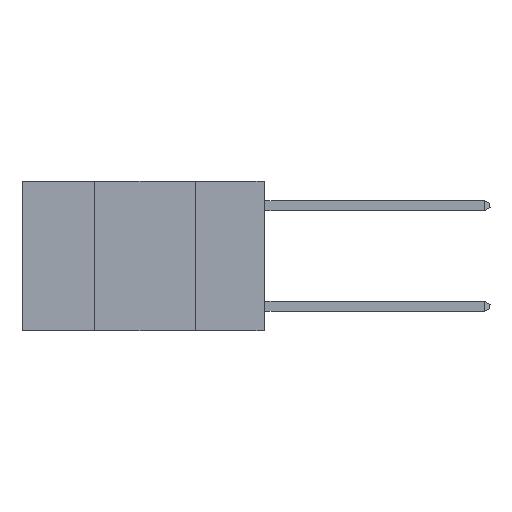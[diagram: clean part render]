
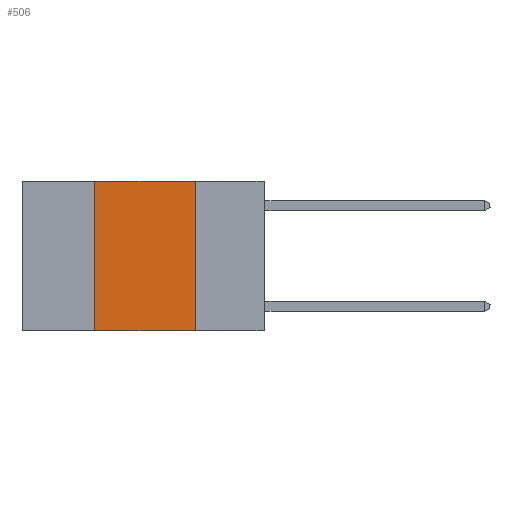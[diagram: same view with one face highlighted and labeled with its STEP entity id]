
A CAD part, left-side view. The second image highlights one B-rep face of the part: STEP entity #506.
In plain terms, the highlighted planar face has unit normal (-1, 0, 0).
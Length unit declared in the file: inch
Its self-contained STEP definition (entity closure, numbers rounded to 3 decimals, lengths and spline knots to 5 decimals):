
#87 = DIRECTION ( 'NONE',  ( 0., -1., 0. ) ) ;
#319 = CARTESIAN_POINT ( 'NONE',  ( 0., 0.42, 0. ) ) ;
#506 = ADVANCED_FACE ( 'NONE', ( #536 ), #17662, .F. ) ;
#536 = FACE_OUTER_BOUND ( 'NONE', #3672, .T. ) ;
#1416 = AXIS2_PLACEMENT_3D ( 'NONE', #10290, #12210, #27448 ) ;
#1519 = EDGE_CURVE ( 'NONE', #7277, #27388, #13245, .T. ) ;
#3672 = EDGE_LOOP ( 'NONE', ( #21942, #30267, #30392, #14577 ) ) ;
#4250 = EDGE_CURVE ( 'NONE', #27388, #6150, #17445, .T. ) ;
#4263 = LINE ( 'NONE', #23806, #19465 ) ;
#5405 = CARTESIAN_POINT ( 'NONE',  ( 0., 0.6, 0. ) ) ;
#6150 = VERTEX_POINT ( 'NONE', #16122 ) ;
#7277 = VERTEX_POINT ( 'NONE', #319 ) ;
#7963 = DIRECTION ( 'NONE',  ( 0., -1., 0. ) ) ;
#10290 = CARTESIAN_POINT ( 'NONE',  ( 0., 0.6, 0. ) ) ;
#12210 = DIRECTION ( 'NONE',  ( 1., 0., 0. ) ) ;
#12755 = CARTESIAN_POINT ( 'NONE',  ( 0., 0.42, -0.37 ) ) ;
#13245 = LINE ( 'NONE', #5405, #14941 ) ;
#13765 = VERTEX_POINT ( 'NONE', #12755 ) ;
#14577 = ORIENTED_EDGE ( 'NONE', *, *, #26245, .T. ) ;
#14941 = VECTOR ( 'NONE', #7963, 39.37008 ) ;
#16122 = CARTESIAN_POINT ( 'NONE',  ( 0., 0.17, -0.37 ) ) ;
#17062 = CARTESIAN_POINT ( 'NONE',  ( 0., 0.6, -0.37 ) ) ;
#17445 = LINE ( 'NONE', #22412, #21580 ) ;
#17662 = PLANE ( 'NONE',  #1416 ) ;
#19465 = VECTOR ( 'NONE', #28471, 39.37008 ) ;
#19943 = LINE ( 'NONE', #17062, #22525 ) ;
#21571 = CARTESIAN_POINT ( 'NONE',  ( 0., 0.17, 0. ) ) ;
#21580 = VECTOR ( 'NONE', #27234, 39.37008 ) ;
#21942 = ORIENTED_EDGE ( 'NONE', *, *, #4250, .F. ) ;
#22412 = CARTESIAN_POINT ( 'NONE',  ( 0., 0.17, 0. ) ) ;
#22525 = VECTOR ( 'NONE', #87, 39.37008 ) ;
#23806 = CARTESIAN_POINT ( 'NONE',  ( 0., 0.42, 0. ) ) ;
#26075 = EDGE_CURVE ( 'NONE', #13765, #7277, #4263, .T. ) ;
#26245 = EDGE_CURVE ( 'NONE', #13765, #6150, #19943, .T. ) ;
#27234 = DIRECTION ( 'NONE',  ( 0., 0., -1. ) ) ;
#27388 = VERTEX_POINT ( 'NONE', #21571 ) ;
#27448 = DIRECTION ( 'NONE',  ( 0., 0., -1. ) ) ;
#28471 = DIRECTION ( 'NONE',  ( 0., 0., 1. ) ) ;
#30267 = ORIENTED_EDGE ( 'NONE', *, *, #1519, .F. ) ;
#30392 = ORIENTED_EDGE ( 'NONE', *, *, #26075, .F. ) ;
